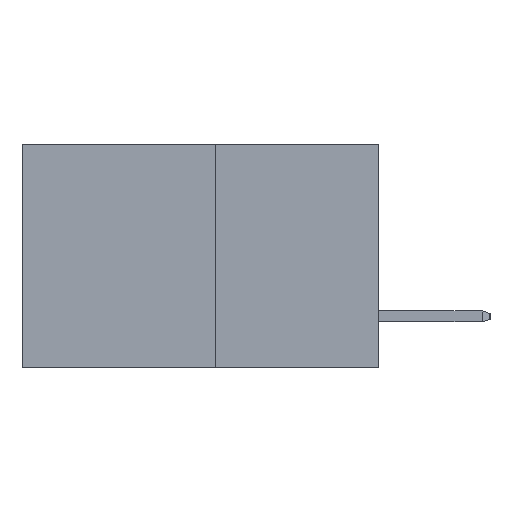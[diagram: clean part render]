
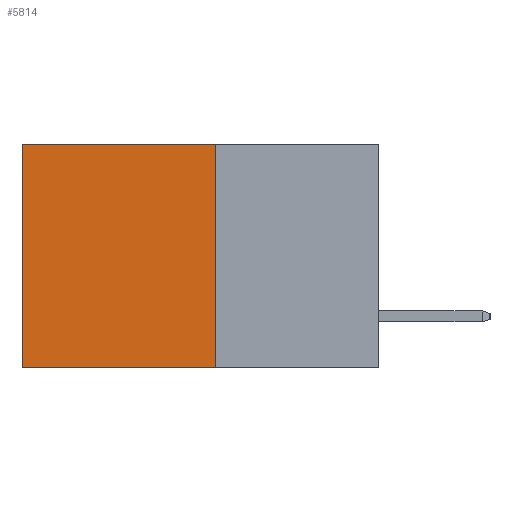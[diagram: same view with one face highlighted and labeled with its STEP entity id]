
A CAD part, left-side view. The second image highlights one B-rep face of the part: STEP entity #5814.
In plain terms, the highlighted planar face has unit normal (-1, 0, 0).
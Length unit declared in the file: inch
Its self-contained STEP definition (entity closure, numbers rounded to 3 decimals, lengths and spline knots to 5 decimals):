
#29 = VECTOR ( 'NONE', #1471, 39.37008 ) ;
#622 = LINE ( 'NONE', #10978, #6207 ) ;
#955 = EDGE_CURVE ( 'NONE', #3362, #13563, #6380, .T. ) ;
#1187 = EDGE_LOOP ( 'NONE', ( #10017, #11719, #1492, #12150 ) ) ;
#1471 = DIRECTION ( 'NONE',  ( 0., 1., 0. ) ) ;
#1492 = ORIENTED_EDGE ( 'NONE', *, *, #955, .F. ) ;
#1977 = FACE_OUTER_BOUND ( 'NONE', #1187, .T. ) ;
#2082 = PLANE ( 'NONE',  #7654 ) ;
#2620 = LINE ( 'NONE', #8129, #29 ) ;
#3046 = CARTESIAN_POINT ( 'NONE',  ( 0.277, 0.27, -0.37 ) ) ;
#3194 = DIRECTION ( 'NONE',  ( 0., 0., -1. ) ) ;
#3362 = VERTEX_POINT ( 'NONE', #12094 ) ;
#3587 = CARTESIAN_POINT ( 'NONE',  ( 0.277, 0.59, -0.37 ) ) ;
#5672 = CARTESIAN_POINT ( 'NONE',  ( 0.277, 0.59, 0. ) ) ;
#5814 = ADVANCED_FACE ( 'NONE', ( #1977 ), #2082, .F. ) ;
#6036 = VERTEX_POINT ( 'NONE', #3587 ) ;
#6207 = VECTOR ( 'NONE', #6509, 39.37008 ) ;
#6284 = LINE ( 'NONE', #13818, #12158 ) ;
#6380 = LINE ( 'NONE', #8933, #9006 ) ;
#6509 = DIRECTION ( 'NONE',  ( 0., 1., 0. ) ) ;
#7654 = AXIS2_PLACEMENT_3D ( 'NONE', #14188, #9874, #3194 ) ;
#8129 = CARTESIAN_POINT ( 'NONE',  ( 0.277, 0.27, -0.37 ) ) ;
#8204 = EDGE_CURVE ( 'NONE', #11959, #6036, #6284, .T. ) ;
#8933 = CARTESIAN_POINT ( 'NONE',  ( 0.277, 0.27, -0.37 ) ) ;
#9006 = VECTOR ( 'NONE', #11931, 39.37008 ) ;
#9487 = DIRECTION ( 'NONE',  ( 0., 0., -1. ) ) ;
#9874 = DIRECTION ( 'NONE',  ( 1., 0., 0. ) ) ;
#9909 = EDGE_CURVE ( 'NONE', #13563, #6036, #2620, .T. ) ;
#10017 = ORIENTED_EDGE ( 'NONE', *, *, #8204, .T. ) ;
#10978 = CARTESIAN_POINT ( 'NONE',  ( 0.277, 0.27, 0. ) ) ;
#11719 = ORIENTED_EDGE ( 'NONE', *, *, #9909, .F. ) ;
#11931 = DIRECTION ( 'NONE',  ( 0., 0., -1. ) ) ;
#11959 = VERTEX_POINT ( 'NONE', #5672 ) ;
#12094 = CARTESIAN_POINT ( 'NONE',  ( 0.277, 0.27, 0. ) ) ;
#12150 = ORIENTED_EDGE ( 'NONE', *, *, #13014, .T. ) ;
#12158 = VECTOR ( 'NONE', #9487, 39.37008 ) ;
#13014 = EDGE_CURVE ( 'NONE', #3362, #11959, #622, .T. ) ;
#13563 = VERTEX_POINT ( 'NONE', #3046 ) ;
#13818 = CARTESIAN_POINT ( 'NONE',  ( 0.277, 0.59, -0.37 ) ) ;
#14188 = CARTESIAN_POINT ( 'NONE',  ( 0.277, 0.27, -0.37 ) ) ;
